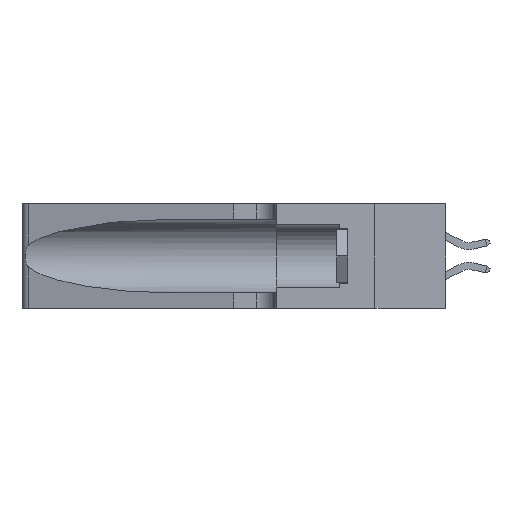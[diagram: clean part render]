
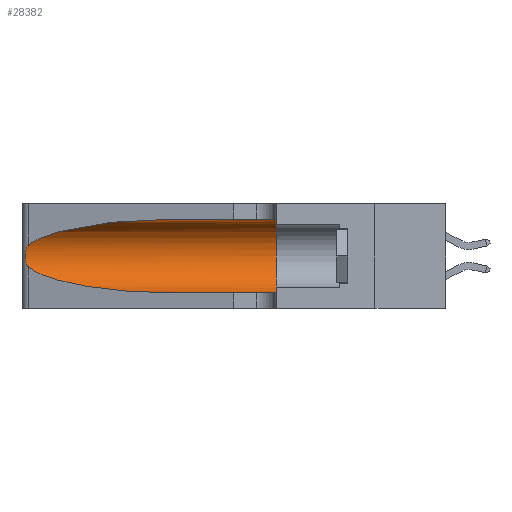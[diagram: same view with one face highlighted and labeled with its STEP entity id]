
A CAD part, left-side view. The second image highlights one B-rep face of the part: STEP entity #28382.
In plain terms, the highlighted cylindrical face has radius 3.308 mm (diameter 6.617 mm), a partial arc.
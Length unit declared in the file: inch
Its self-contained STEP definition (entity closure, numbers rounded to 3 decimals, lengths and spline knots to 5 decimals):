
#61 = DIRECTION ( 'NONE',  ( 0., 0., 1. ) ) ;
#2016 = CARTESIAN_POINT ( 'NONE',  ( 0.25639, 1.23186, 0.15144 ) ) ;
#2469 = CARTESIAN_POINT ( 'NONE',  ( 0.1305, 0.72297, 0.31525 ) ) ;
#3356 = DIRECTION ( 'NONE',  ( 0., 0., -1. ) ) ;
#4013 =( BOUNDED_CURVE ( )  B_SPLINE_CURVE ( 3, ( #25844, #4238, #10453, #32025 ),
 .UNSPECIFIED., .F., .F. ) 
 B_SPLINE_CURVE_WITH_KNOTS ( ( 4, 4 ),
 ( 3.44316, 4.71239 ),
 .UNSPECIFIED. ) 
 CURVE ( )  GEOMETRIC_REPRESENTATION_ITEM ( )  RATIONAL_B_SPLINE_CURVE ( ( 1., 0.87, 0.87, 1. ) ) 
 REPRESENTATION_ITEM ( '' )  );
#4111 = EDGE_CURVE ( 'NONE', #36281, #30412, #14696, .T. ) ;
#4238 = CARTESIAN_POINT ( 'NONE',  ( 0.2373, 1.15595, 0.08982 ) ) ;
#4499 = AXIS2_PLACEMENT_3D ( 'NONE', #34235, #28061, #3356 ) ;
#4980 = CARTESIAN_POINT ( 'NONE',  ( 0.25487, 1.22718, 0.22369 ) ) ;
#5117 = CARTESIAN_POINT ( 'NONE',  ( 0.25487, 1.22718, 0.14631 ) ) ;
#5569 = CARTESIAN_POINT ( 'NONE',  ( 0.18966, 0.96281, 0.31525 ) ) ;
#6384 = ORIENTED_EDGE ( 'NONE', *, *, #15339, .T. ) ;
#8089 = CARTESIAN_POINT ( 'NONE',  ( 0.25639, 1.23184, 0.21858 ) ) ;
#8679 = CARTESIAN_POINT ( 'NONE',  ( 0.25487, 1.22718, 0.22369 ) ) ;
#9536 = CARTESIAN_POINT ( 'NONE',  ( 0.1305, 0.35, 0.31525 ) ) ;
#9685 = CARTESIAN_POINT ( 'NONE',  ( 0.1305, 1.61858, 0.31525 ) ) ;
#10453 = CARTESIAN_POINT ( 'NONE',  ( 0.18966, 0.96281, 0.05475 ) ) ;
#11215 = CARTESIAN_POINT ( 'NONE',  ( 0.25854, 1.2359, 0.20912 ) ) ;
#11343 = CARTESIAN_POINT ( 'NONE',  ( 0.1305, 0.72297, 0.31525 ) ) ;
#12948 = VERTEX_POINT ( 'NONE', #26096 ) ;
#13721 = VECTOR ( 'NONE', #28176, 39.37008 ) ;
#14176 = CARTESIAN_POINT ( 'NONE',  ( 0.25555, 1.22994, 0.2215 ) ) ;
#14313 = CARTESIAN_POINT ( 'NONE',  ( 0.26075, 1.23896, 0.19203 ) ) ;
#14334 = VECTOR ( 'NONE', #38057, 39.37008 ) ;
#14696 = LINE ( 'NONE', #9685, #13721 ) ;
#15339 = EDGE_CURVE ( 'NONE', #23815, #30877, #23524, .T. ) ;
#15949 = CYLINDRICAL_SURFACE ( 'NONE', #4499, 0.13025 ) ;
#16897 = FACE_OUTER_BOUND ( 'NONE', #29553, .T. ) ;
#17341 = ORIENTED_EDGE ( 'NONE', *, *, #27210, .T. ) ;
#17415 = CARTESIAN_POINT ( 'NONE',  ( 0.26017, 1.23833, 0.17102 ) ) ;
#17565 = ORIENTED_EDGE ( 'NONE', *, *, #34211, .F. ) ;
#18561 = DIRECTION ( 'NONE',  ( 0., 1., 0. ) ) ;
#18568 = ORIENTED_EDGE ( 'NONE', *, *, #29962, .T. ) ;
#19137 = ORIENTED_EDGE ( 'NONE', *, *, #27511, .T. ) ;
#20541 = CARTESIAN_POINT ( 'NONE',  ( 0.25789, 1.23486, 0.15765 ) ) ;
#22610 = CARTESIAN_POINT ( 'NONE',  ( 0.1305, 1.61858, 0.05475 ) ) ;
#23524 = LINE ( 'NONE', #22610, #14334 ) ;
#23633 = CARTESIAN_POINT ( 'NONE',  ( 0.25555, 1.22993, 0.14849 ) ) ;
#23815 = VERTEX_POINT ( 'NONE', #36921 ) ;
#24009 = CIRCLE ( 'NONE', #38250, 0.13025 ) ;
#25844 = CARTESIAN_POINT ( 'NONE',  ( 0.25487, 1.22718, 0.14631 ) ) ;
#26096 = CARTESIAN_POINT ( 'NONE',  ( 0.25487, 1.22718, 0.14631 ) ) ;
#27181 = CARTESIAN_POINT ( 'NONE',  ( 0.2373, 1.15595, 0.28018 ) ) ;
#27187 = VERTEX_POINT ( 'NONE', #28674 ) ;
#27210 = EDGE_CURVE ( 'NONE', #12948, #23815, #4013, .T. ) ;
#27511 = EDGE_CURVE ( 'NONE', #36281, #27187, #36890, .T. ) ;
#28061 = DIRECTION ( 'NONE',  ( 0., -1., 0. ) ) ;
#28176 = DIRECTION ( 'NONE',  ( 0., -1., 0. ) ) ;
#28382 = ADVANCED_FACE ( 'NONE', ( #16897 ), #15949, .F. ) ;
#28674 = CARTESIAN_POINT ( 'NONE',  ( 0.25487, 1.22718, 0.22369 ) ) ;
#29553 = EDGE_LOOP ( 'NONE', ( #19137, #18568, #17341, #6384, #17565, #29736 ) ) ;
#29660 = CARTESIAN_POINT ( 'NONE',  ( 0.25787, 1.23484, 0.2124 ) ) ;
#29709 = B_SPLINE_CURVE_WITH_KNOTS ( 'NONE', 3,
 ( #4980, #14176, #8089, #29660, #11215, #32796, #14313, #35892, #17415, #38963, #20541, #2016, #23633, #5117 ),
 .UNSPECIFIED., .F., .F.,
 ( 4, 2, 2, 2, 2, 2, 4 ),
 ( 0., 0.00027, 0.00053, 0.00107, 0.0016, 0.00187, 0.00214 ),
 .UNSPECIFIED. ) ;
#29736 = ORIENTED_EDGE ( 'NONE', *, *, #4111, .F. ) ;
#29962 = EDGE_CURVE ( 'NONE', #27187, #12948, #29709, .T. ) ;
#30412 = VERTEX_POINT ( 'NONE', #9536 ) ;
#30877 = VERTEX_POINT ( 'NONE', #33096 ) ;
#32025 = CARTESIAN_POINT ( 'NONE',  ( 0.1305, 0.72297, 0.05475 ) ) ;
#32796 = CARTESIAN_POINT ( 'NONE',  ( 0.26018, 1.23835, 0.19895 ) ) ;
#33096 = CARTESIAN_POINT ( 'NONE',  ( 0.1305, 0.35, 0.05475 ) ) ;
#34211 = EDGE_CURVE ( 'NONE', #30412, #30877, #24009, .T. ) ;
#34235 = CARTESIAN_POINT ( 'NONE',  ( 0.1305, 1.61858, 0.185 ) ) ;
#35892 = CARTESIAN_POINT ( 'NONE',  ( 0.26075, 1.23896, 0.178 ) ) ;
#36281 = VERTEX_POINT ( 'NONE', #11343 ) ;
#36890 =( BOUNDED_CURVE ( )  B_SPLINE_CURVE ( 3, ( #2469, #5569, #27181, #8679 ),
 .UNSPECIFIED., .F., .F. ) 
 B_SPLINE_CURVE_WITH_KNOTS ( ( 4, 4 ),
 ( 1.5708, 2.84003 ),
 .UNSPECIFIED. ) 
 CURVE ( )  GEOMETRIC_REPRESENTATION_ITEM ( )  RATIONAL_B_SPLINE_CURVE ( ( 1., 0.87, 0.87, 1. ) ) 
 REPRESENTATION_ITEM ( '' )  );
#36921 = CARTESIAN_POINT ( 'NONE',  ( 0.1305, 0.72297, 0.05475 ) ) ;
#36990 = CARTESIAN_POINT ( 'NONE',  ( 0.1305, 0.35, 0.185 ) ) ;
#38057 = DIRECTION ( 'NONE',  ( 0., -1., 0. ) ) ;
#38250 = AXIS2_PLACEMENT_3D ( 'NONE', #36990, #18561, #61 ) ;
#38963 = CARTESIAN_POINT ( 'NONE',  ( 0.25856, 1.23593, 0.16098 ) ) ;
